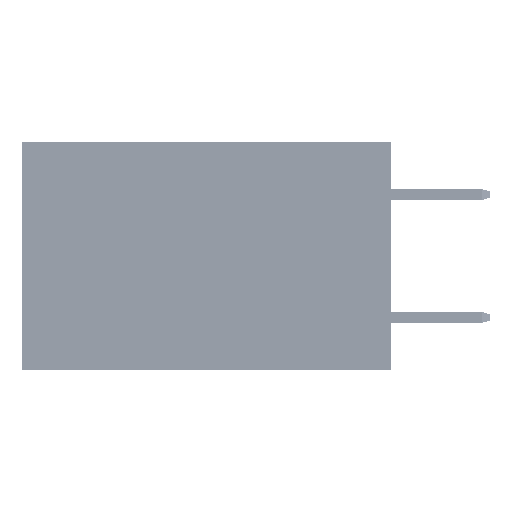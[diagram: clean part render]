
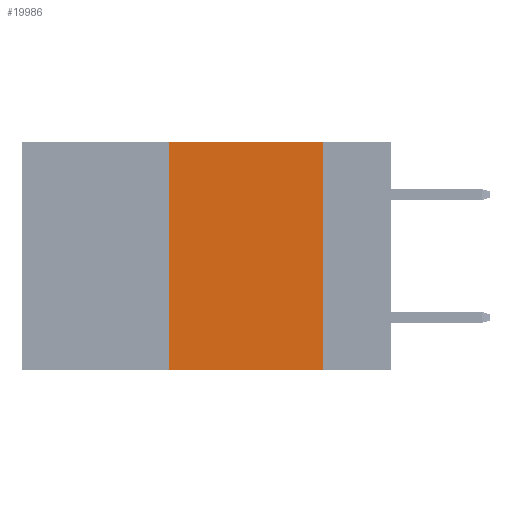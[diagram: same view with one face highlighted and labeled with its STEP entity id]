
A CAD part, left-side view. The second image highlights one B-rep face of the part: STEP entity #19986.
In plain terms, the highlighted planar face has unit normal (-1, 0, 0).
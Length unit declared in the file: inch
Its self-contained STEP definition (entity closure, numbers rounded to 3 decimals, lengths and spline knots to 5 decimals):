
#3196 = EDGE_CURVE ( 'NONE', #35399, #22997, #41880, .T. ) ;
#4890 = AXIS2_PLACEMENT_3D ( 'NONE', #14552, #41525, #18472 ) ;
#5640 = ORIENTED_EDGE ( 'NONE', *, *, #15518, .F. ) ;
#6077 = FACE_OUTER_BOUND ( 'NONE', #32374, .T. ) ;
#7097 = DIRECTION ( 'NONE',  ( 0., -1., 0. ) ) ;
#7511 = VECTOR ( 'NONE', #43248, 39.37008 ) ;
#11417 = CARTESIAN_POINT ( 'NONE',  ( 0., 0.6, 0. ) ) ;
#12931 = VERTEX_POINT ( 'NONE', #40815 ) ;
#14552 = CARTESIAN_POINT ( 'NONE',  ( 0., 0.6, 0. ) ) ;
#15518 = EDGE_CURVE ( 'NONE', #12931, #27931, #29831, .T. ) ;
#16308 = CARTESIAN_POINT ( 'NONE',  ( 0., 0.36, 0. ) ) ;
#17973 = LINE ( 'NONE', #16308, #7511 ) ;
#18472 = DIRECTION ( 'NONE',  ( 0., 0., -1. ) ) ;
#18589 = ORIENTED_EDGE ( 'NONE', *, *, #44378, .F. ) ;
#19986 = ADVANCED_FACE ( 'NONE', ( #6077 ), #29937, .F. ) ;
#22790 = DIRECTION ( 'NONE',  ( 0., 0., -1. ) ) ;
#22841 = EDGE_CURVE ( 'NONE', #27931, #22997, #46931, .T. ) ;
#22951 = DIRECTION ( 'NONE',  ( 0., -1., 0. ) ) ;
#22997 = VERTEX_POINT ( 'NONE', #27481 ) ;
#25058 = CARTESIAN_POINT ( 'NONE',  ( 0., 0.11, 0. ) ) ;
#27157 = CARTESIAN_POINT ( 'NONE',  ( 0., 0.36, -0.37 ) ) ;
#27481 = CARTESIAN_POINT ( 'NONE',  ( 0., 0.11, -0.37 ) ) ;
#27931 = VERTEX_POINT ( 'NONE', #25058 ) ;
#29831 = LINE ( 'NONE', #11417, #50021 ) ;
#29937 = PLANE ( 'NONE',  #4890 ) ;
#30471 = VECTOR ( 'NONE', #7097, 39.37008 ) ;
#32374 = EDGE_LOOP ( 'NONE', ( #42642, #5640, #18589, #33041 ) ) ;
#33041 = ORIENTED_EDGE ( 'NONE', *, *, #3196, .T. ) ;
#34275 = CARTESIAN_POINT ( 'NONE',  ( 0., 0.11, 0. ) ) ;
#34300 = CARTESIAN_POINT ( 'NONE',  ( 0., 0.6, -0.37 ) ) ;
#35399 = VERTEX_POINT ( 'NONE', #27157 ) ;
#40815 = CARTESIAN_POINT ( 'NONE',  ( 0., 0.36, 0. ) ) ;
#41525 = DIRECTION ( 'NONE',  ( 1., 0., 0. ) ) ;
#41880 = LINE ( 'NONE', #34300, #30471 ) ;
#42642 = ORIENTED_EDGE ( 'NONE', *, *, #22841, .F. ) ;
#43248 = DIRECTION ( 'NONE',  ( 0., 0., 1. ) ) ;
#44378 = EDGE_CURVE ( 'NONE', #35399, #12931, #17973, .T. ) ;
#45777 = VECTOR ( 'NONE', #22790, 39.37008 ) ;
#46931 = LINE ( 'NONE', #34275, #45777 ) ;
#50021 = VECTOR ( 'NONE', #22951, 39.37008 ) ;
